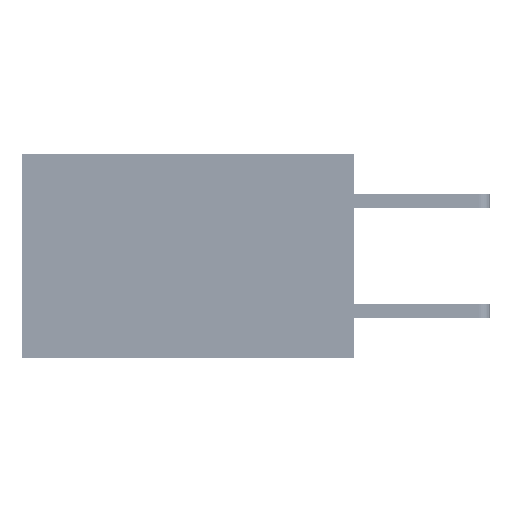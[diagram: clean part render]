
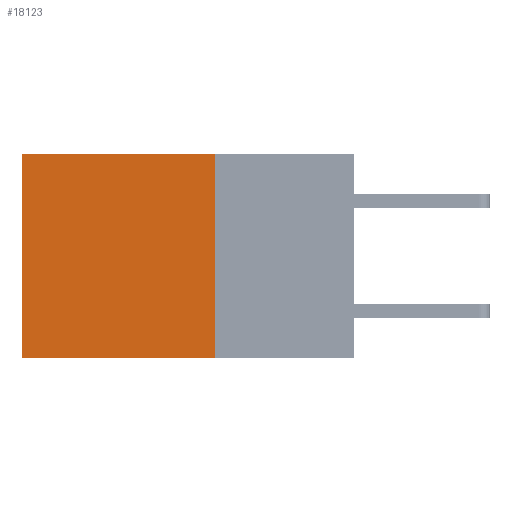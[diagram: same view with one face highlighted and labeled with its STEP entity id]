
A CAD part, left-side view. The second image highlights one B-rep face of the part: STEP entity #18123.
In plain terms, the highlighted planar face has unit normal (-1, 0, 0).
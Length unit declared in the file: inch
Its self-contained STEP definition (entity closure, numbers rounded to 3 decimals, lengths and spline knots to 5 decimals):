
#1394 = EDGE_CURVE ( 'NONE', #13996, #1555, #9066, .T. ) ;
#1555 = VERTEX_POINT ( 'NONE', #23294 ) ;
#1918 = PLANE ( 'NONE',  #41858 ) ;
#3165 = ORIENTED_EDGE ( 'NONE', *, *, #1394, .T. ) ;
#5431 = CARTESIAN_POINT ( 'NONE',  ( 0.2875, 0.6, 0. ) ) ;
#6267 = ORIENTED_EDGE ( 'NONE', *, *, #14126, .F. ) ;
#6811 = VECTOR ( 'NONE', #24341, 39.37008 ) ;
#9066 = LINE ( 'NONE', #5431, #6811 ) ;
#9277 = ORIENTED_EDGE ( 'NONE', *, *, #45747, .T. ) ;
#13562 = EDGE_LOOP ( 'NONE', ( #3165, #6267, #21559, #9277 ) ) ;
#13996 = VERTEX_POINT ( 'NONE', #40589 ) ;
#14126 = EDGE_CURVE ( 'NONE', #39704, #1555, #23837, .T. ) ;
#14519 = CARTESIAN_POINT ( 'NONE',  ( 0.2875, 0.25, 0. ) ) ;
#15380 = CARTESIAN_POINT ( 'NONE',  ( 0.2875, 0.25, -0.37 ) ) ;
#15563 = DIRECTION ( 'NONE',  ( 0., 0., -1. ) ) ;
#16419 = FACE_OUTER_BOUND ( 'NONE', #13562, .T. ) ;
#16485 = DIRECTION ( 'NONE',  ( 0., 1., 0. ) ) ;
#16734 = LINE ( 'NONE', #20830, #45385 ) ;
#18123 = ADVANCED_FACE ( 'NONE', ( #16419 ), #1918, .F. ) ;
#20830 = CARTESIAN_POINT ( 'NONE',  ( 0.2875, 0.25, 0. ) ) ;
#21559 = ORIENTED_EDGE ( 'NONE', *, *, #42957, .F. ) ;
#23294 = CARTESIAN_POINT ( 'NONE',  ( 0.2875, 0.6, -0.37 ) ) ;
#23837 = LINE ( 'NONE', #24072, #30114 ) ;
#24072 = CARTESIAN_POINT ( 'NONE',  ( 0.2875, 0.25, -0.37 ) ) ;
#24324 = DIRECTION ( 'NONE',  ( 0., 1., 0. ) ) ;
#24341 = DIRECTION ( 'NONE',  ( 0., 0., -1. ) ) ;
#27511 = VERTEX_POINT ( 'NONE', #14519 ) ;
#30114 = VECTOR ( 'NONE', #24324, 39.37008 ) ;
#31236 = DIRECTION ( 'NONE',  ( 1., 0., 0. ) ) ;
#33299 = LINE ( 'NONE', #34002, #38991 ) ;
#34002 = CARTESIAN_POINT ( 'NONE',  ( 0.2875, 0.25, 0. ) ) ;
#34380 = CARTESIAN_POINT ( 'NONE',  ( 0.2875, 0.25, 0. ) ) ;
#38991 = VECTOR ( 'NONE', #15563, 39.37008 ) ;
#39704 = VERTEX_POINT ( 'NONE', #15380 ) ;
#40589 = CARTESIAN_POINT ( 'NONE',  ( 0.2875, 0.6, 0. ) ) ;
#41858 = AXIS2_PLACEMENT_3D ( 'NONE', #34380, #31236, #46012 ) ;
#42957 = EDGE_CURVE ( 'NONE', #27511, #39704, #33299, .T. ) ;
#45385 = VECTOR ( 'NONE', #16485, 39.37008 ) ;
#45747 = EDGE_CURVE ( 'NONE', #27511, #13996, #16734, .T. ) ;
#46012 = DIRECTION ( 'NONE',  ( 0., 0., -1. ) ) ;
